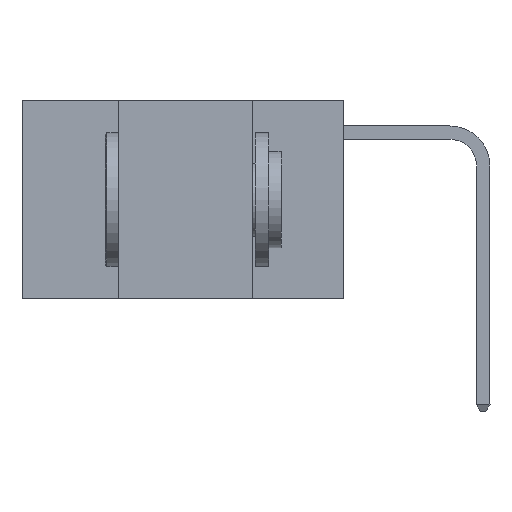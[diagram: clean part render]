
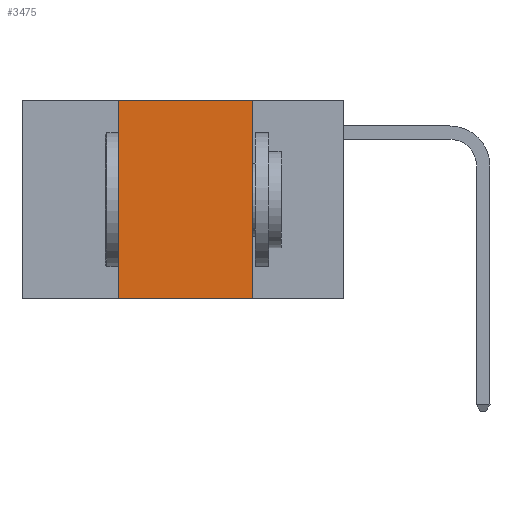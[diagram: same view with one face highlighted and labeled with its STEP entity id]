
A CAD part, left-side view. The second image highlights one B-rep face of the part: STEP entity #3475.
In plain terms, the highlighted planar face has unit normal (-1, 0, 0).
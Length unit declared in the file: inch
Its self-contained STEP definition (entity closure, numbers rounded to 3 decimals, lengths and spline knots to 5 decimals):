
#62 = FACE_OUTER_BOUND ( 'NONE', #9232, .T. ) ;
#274 = ORIENTED_EDGE ( 'NONE', *, *, #5942, .F. ) ;
#297 = EDGE_CURVE ( 'NONE', #3736, #10091, #2430, .T. ) ;
#1006 = DIRECTION ( 'NONE',  ( 0., -1., 0. ) ) ;
#1076 = VECTOR ( 'NONE', #1006, 39.37008 ) ;
#1336 = ORIENTED_EDGE ( 'NONE', *, *, #297, .F. ) ;
#1640 = CARTESIAN_POINT ( 'NONE',  ( 0., 0.42, 0. ) ) ;
#1839 = EDGE_CURVE ( 'NONE', #9251, #10091, #2520, .T. ) ;
#2242 = LINE ( 'NONE', #5728, #1076 ) ;
#2430 = LINE ( 'NONE', #3197, #5362 ) ;
#2520 = LINE ( 'NONE', #7809, #6136 ) ;
#2707 = VECTOR ( 'NONE', #7776, 39.37008 ) ;
#3197 = CARTESIAN_POINT ( 'NONE',  ( 0., 0.17, 0. ) ) ;
#3380 = CARTESIAN_POINT ( 'NONE',  ( 0., 0.6, 0. ) ) ;
#3475 = ADVANCED_FACE ( 'NONE', ( #62 ), #9542, .F. ) ;
#3535 = DIRECTION ( 'NONE',  ( 1., 0., 0. ) ) ;
#3736 = VERTEX_POINT ( 'NONE', #5571 ) ;
#4169 = DIRECTION ( 'NONE',  ( 0., 0., -1. ) ) ;
#5362 = VECTOR ( 'NONE', #4169, 39.37008 ) ;
#5571 = CARTESIAN_POINT ( 'NONE',  ( 0., 0.17, 0. ) ) ;
#5586 = CARTESIAN_POINT ( 'NONE',  ( 0., 0.42, 0. ) ) ;
#5728 = CARTESIAN_POINT ( 'NONE',  ( 0., 0.6, 0. ) ) ;
#5942 = EDGE_CURVE ( 'NONE', #9349, #3736, #2242, .T. ) ;
#6008 = DIRECTION ( 'NONE',  ( 0., -1., 0. ) ) ;
#6136 = VECTOR ( 'NONE', #6008, 39.37008 ) ;
#6518 = AXIS2_PLACEMENT_3D ( 'NONE', #3380, #3535, #11304 ) ;
#7451 = ORIENTED_EDGE ( 'NONE', *, *, #1839, .T. ) ;
#7593 = EDGE_CURVE ( 'NONE', #9251, #9349, #9520, .T. ) ;
#7776 = DIRECTION ( 'NONE',  ( 0., 0., 1. ) ) ;
#7809 = CARTESIAN_POINT ( 'NONE',  ( 0., 0.6, -0.37 ) ) ;
#7903 = ORIENTED_EDGE ( 'NONE', *, *, #7593, .F. ) ;
#7993 = CARTESIAN_POINT ( 'NONE',  ( 0., 0.17, -0.37 ) ) ;
#9232 = EDGE_LOOP ( 'NONE', ( #1336, #274, #7903, #7451 ) ) ;
#9251 = VERTEX_POINT ( 'NONE', #9723 ) ;
#9349 = VERTEX_POINT ( 'NONE', #5586 ) ;
#9520 = LINE ( 'NONE', #1640, #2707 ) ;
#9542 = PLANE ( 'NONE',  #6518 ) ;
#9723 = CARTESIAN_POINT ( 'NONE',  ( 0., 0.42, -0.37 ) ) ;
#10091 = VERTEX_POINT ( 'NONE', #7993 ) ;
#11304 = DIRECTION ( 'NONE',  ( 0., 0., -1. ) ) ;
